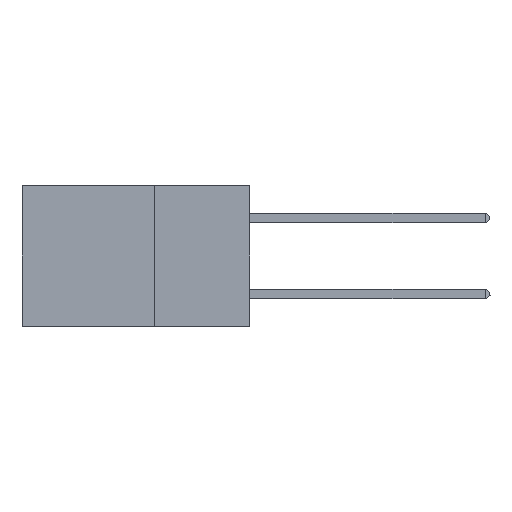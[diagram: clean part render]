
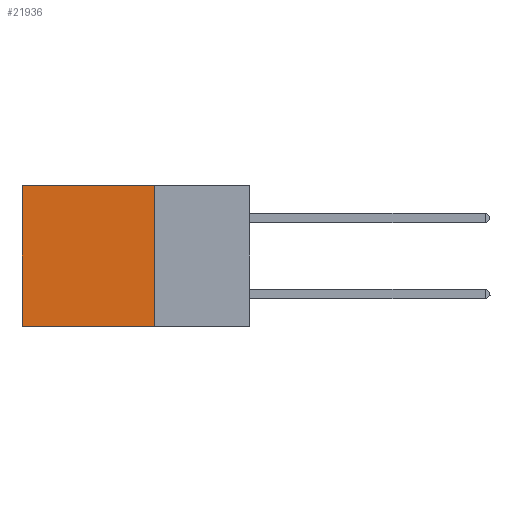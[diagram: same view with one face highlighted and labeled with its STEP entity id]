
A CAD part, left-side view. The second image highlights one B-rep face of the part: STEP entity #21936.
In plain terms, the highlighted planar face has unit normal (-1, 0, 0).
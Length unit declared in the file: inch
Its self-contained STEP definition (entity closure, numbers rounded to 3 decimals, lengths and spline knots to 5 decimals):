
#716 = VECTOR ( 'NONE', #3375, 39.37008 ) ;
#858 = VERTEX_POINT ( 'NONE', #6537 ) ;
#1878 = EDGE_CURVE ( 'NONE', #7938, #12971, #17474, .T. ) ;
#2716 = CARTESIAN_POINT ( 'NONE',  ( 0.2875, 0.25, 0. ) ) ;
#3375 = DIRECTION ( 'NONE',  ( 0., 1., 0. ) ) ;
#4365 = ORIENTED_EDGE ( 'NONE', *, *, #1878, .T. ) ;
#4937 = VECTOR ( 'NONE', #17581, 39.37008 ) ;
#5203 = FACE_OUTER_BOUND ( 'NONE', #18925, .T. ) ;
#5922 = LINE ( 'NONE', #23678, #17830 ) ;
#6537 = CARTESIAN_POINT ( 'NONE',  ( 0.2875, 0.25, -0.37 ) ) ;
#6595 = DIRECTION ( 'NONE',  ( 1., 0., 0. ) ) ;
#7019 = CARTESIAN_POINT ( 'NONE',  ( 0.2875, 0.6, -0.37 ) ) ;
#7173 = CARTESIAN_POINT ( 'NONE',  ( 0.2875, 0.6, 0. ) ) ;
#7938 = VERTEX_POINT ( 'NONE', #2716 ) ;
#9219 = ORIENTED_EDGE ( 'NONE', *, *, #21431, .F. ) ;
#10559 = LINE ( 'NONE', #19947, #4937 ) ;
#12971 = VERTEX_POINT ( 'NONE', #7173 ) ;
#14207 = EDGE_CURVE ( 'NONE', #7938, #858, #5922, .T. ) ;
#14997 = DIRECTION ( 'NONE',  ( 0., 0., -1. ) ) ;
#15459 = VECTOR ( 'NONE', #20413, 39.37008 ) ;
#15489 = DIRECTION ( 'NONE',  ( 0., 0., -1. ) ) ;
#15497 = VERTEX_POINT ( 'NONE', #7019 ) ;
#15988 = CARTESIAN_POINT ( 'NONE',  ( 0.2875, 0.25, 0. ) ) ;
#16835 = AXIS2_PLACEMENT_3D ( 'NONE', #21142, #6595, #14997 ) ;
#17474 = LINE ( 'NONE', #15988, #716 ) ;
#17581 = DIRECTION ( 'NONE',  ( 0., 0., -1. ) ) ;
#17830 = VECTOR ( 'NONE', #15489, 39.37008 ) ;
#17946 = ORIENTED_EDGE ( 'NONE', *, *, #25955, .T. ) ;
#18925 = EDGE_LOOP ( 'NONE', ( #17946, #9219, #25032, #4365 ) ) ;
#19947 = CARTESIAN_POINT ( 'NONE',  ( 0.2875, 0.6, 0. ) ) ;
#20413 = DIRECTION ( 'NONE',  ( 0., 1., 0. ) ) ;
#21142 = CARTESIAN_POINT ( 'NONE',  ( 0.2875, 0.25, 0. ) ) ;
#21226 = PLANE ( 'NONE',  #16835 ) ;
#21431 = EDGE_CURVE ( 'NONE', #858, #15497, #21668, .T. ) ;
#21668 = LINE ( 'NONE', #24913, #15459 ) ;
#21936 = ADVANCED_FACE ( 'NONE', ( #5203 ), #21226, .F. ) ;
#23678 = CARTESIAN_POINT ( 'NONE',  ( 0.2875, 0.25, 0. ) ) ;
#24913 = CARTESIAN_POINT ( 'NONE',  ( 0.2875, 0.25, -0.37 ) ) ;
#25032 = ORIENTED_EDGE ( 'NONE', *, *, #14207, .F. ) ;
#25955 = EDGE_CURVE ( 'NONE', #12971, #15497, #10559, .T. ) ;
